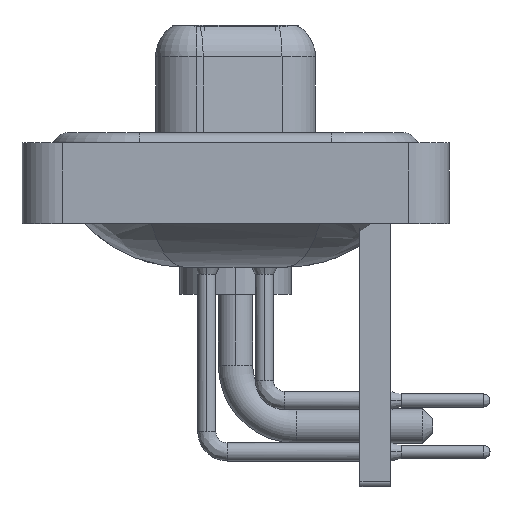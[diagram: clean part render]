
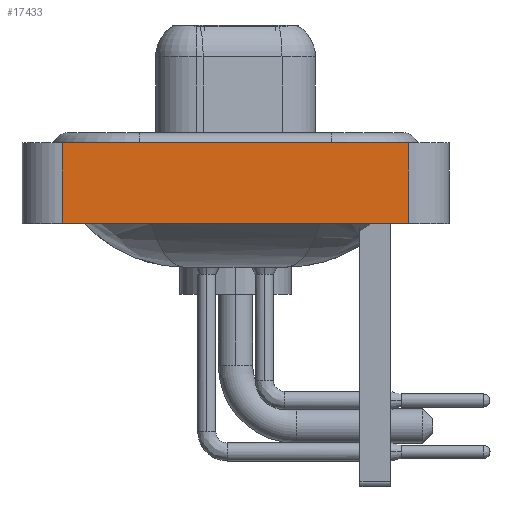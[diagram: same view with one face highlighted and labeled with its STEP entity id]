
A CAD part, left-side view. The second image highlights one B-rep face of the part: STEP entity #17433.
In plain terms, the highlighted planar face has unit normal (-1, 0, 0).
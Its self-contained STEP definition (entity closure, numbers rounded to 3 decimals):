
#634 = ORIENTED_EDGE ( 'NONE', *, *, #26237, .T. ) ;
#1342 = EDGE_LOOP ( 'NONE', ( #634, #15869, #21035, #3707 ) ) ;
#1363 = DIRECTION ( 'NONE',  ( 0., 0., 1. ) ) ;
#1641 = CARTESIAN_POINT ( 'NONE',  ( -7.35, -8.55, -3.6 ) ) ;
#1914 = EDGE_CURVE ( 'NONE', #23672, #26219, #6905, .T. ) ;
#1940 = VERTEX_POINT ( 'NONE', #13522 ) ;
#2180 = EDGE_CURVE ( 'NONE', #1940, #23672, #5813, .T. ) ;
#3707 = ORIENTED_EDGE ( 'NONE', *, *, #20862, .T. ) ;
#3724 = VECTOR ( 'NONE', #17398, 1000. ) ;
#3763 = DIRECTION ( 'NONE',  ( 0., 0., 1. ) ) ;
#5085 = AXIS2_PLACEMENT_3D ( 'NONE', #1641, #10348, #1363 ) ;
#5813 = LINE ( 'NONE', #26790, #20027 ) ;
#6905 = LINE ( 'NONE', #15455, #3724 ) ;
#7861 = FACE_OUTER_BOUND ( 'NONE', #1342, .T. ) ;
#8460 = VECTOR ( 'NONE', #25613, 1000. ) ;
#8514 = LINE ( 'NONE', #23396, #8460 ) ;
#9783 = LINE ( 'NONE', #14191, #14704 ) ;
#10348 = DIRECTION ( 'NONE',  ( -1., 0., 0. ) ) ;
#10562 = CARTESIAN_POINT ( 'NONE',  ( -7.35, -8.55, -3.6 ) ) ;
#12279 = PLANE ( 'NONE',  #5085 ) ;
#12577 = VERTEX_POINT ( 'NONE', #10562 ) ;
#12787 = CARTESIAN_POINT ( 'NONE',  ( -7.35, 8.55, 0.4 ) ) ;
#13522 = CARTESIAN_POINT ( 'NONE',  ( -7.35, 8.55, -3.6 ) ) ;
#14191 = CARTESIAN_POINT ( 'NONE',  ( -7.35, -8.55, -3.6 ) ) ;
#14704 = VECTOR ( 'NONE', #22874, 1000. ) ;
#14735 = CARTESIAN_POINT ( 'NONE',  ( -7.35, -8.55, 0.4 ) ) ;
#15455 = CARTESIAN_POINT ( 'NONE',  ( -7.35, -8.55, 0.4 ) ) ;
#15869 = ORIENTED_EDGE ( 'NONE', *, *, #1914, .F. ) ;
#17398 = DIRECTION ( 'NONE',  ( 0., -1., 0. ) ) ;
#17433 = ADVANCED_FACE ( 'NONE', ( #7861 ), #12279, .T. ) ;
#20027 = VECTOR ( 'NONE', #3763, 1000. ) ;
#20862 = EDGE_CURVE ( 'NONE', #1940, #12577, #9783, .T. ) ;
#21035 = ORIENTED_EDGE ( 'NONE', *, *, #2180, .F. ) ;
#22874 = DIRECTION ( 'NONE',  ( 0., -1., 0. ) ) ;
#23396 = CARTESIAN_POINT ( 'NONE',  ( -7.35, -8.55, -3.6 ) ) ;
#23672 = VERTEX_POINT ( 'NONE', #12787 ) ;
#25613 = DIRECTION ( 'NONE',  ( 0., 0., 1. ) ) ;
#26219 = VERTEX_POINT ( 'NONE', #14735 ) ;
#26237 = EDGE_CURVE ( 'NONE', #12577, #26219, #8514, .T. ) ;
#26790 = CARTESIAN_POINT ( 'NONE',  ( -7.35, 8.55, -3.6 ) ) ;
